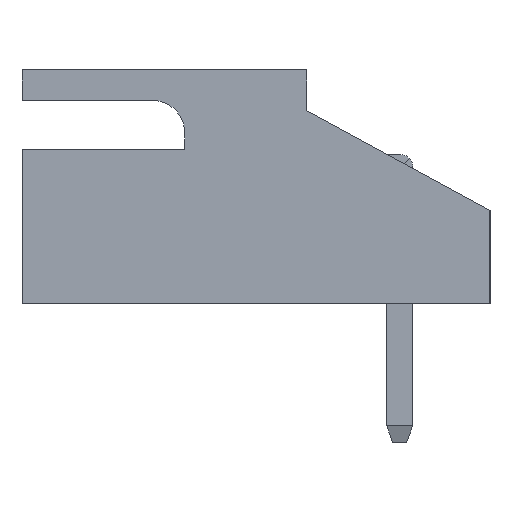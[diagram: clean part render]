
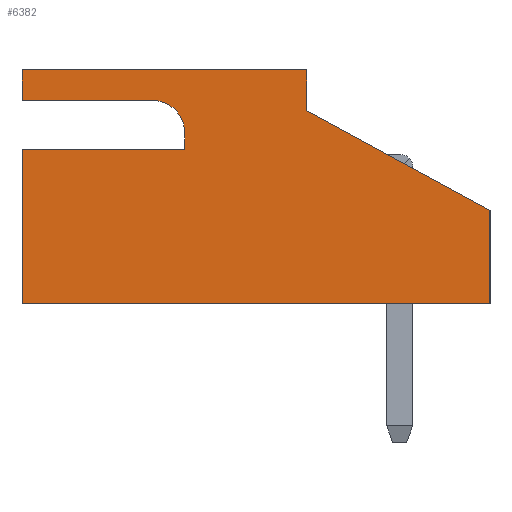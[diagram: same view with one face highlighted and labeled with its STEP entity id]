
A CAD part, left-side view. The second image highlights one B-rep face of the part: STEP entity #6382.
In plain terms, the highlighted planar face has unit normal (-1, 0, 0).
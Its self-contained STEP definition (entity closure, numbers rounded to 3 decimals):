
#104 = LINE ( 'NONE', #4746, #4784 ) ;
#234 = ORIENTED_EDGE ( 'NONE', *, *, #6420, .F. ) ;
#254 = LINE ( 'NONE', #6606, #1631 ) ;
#255 = VERTEX_POINT ( 'NONE', #4761 ) ;
#322 = ORIENTED_EDGE ( 'NONE', *, *, #5219, .T. ) ;
#358 = CARTESIAN_POINT ( 'NONE',  ( -16.25, 7., 0.925 ) ) ;
#362 = LINE ( 'NONE', #5617, #2933 ) ;
#395 = DIRECTION ( 'NONE',  ( 0., 0., -1. ) ) ;
#410 = DIRECTION ( 'NONE',  ( 1., 0., 0. ) ) ;
#445 = CARTESIAN_POINT ( 'NONE',  ( -16.25, 3.8, 1.325 ) ) ;
#536 = LINE ( 'NONE', #4723, #3891 ) ;
#648 = EDGE_CURVE ( 'NONE', #5474, #1851, #536, .T. ) ;
#1144 = CARTESIAN_POINT ( 'NONE',  ( -16.25, 7., 2.875 ) ) ;
#1180 = CARTESIAN_POINT ( 'NONE',  ( -16.25, 3., 0.925 ) ) ;
#1228 = VECTOR ( 'NONE', #1668, 1000. ) ;
#1345 = VERTEX_POINT ( 'NONE', #1497 ) ;
#1456 = LINE ( 'NONE', #6197, #3584 ) ;
#1497 = CARTESIAN_POINT ( 'NONE',  ( -16.25, 3.8, 2.125 ) ) ;
#1550 = VERTEX_POINT ( 'NONE', #6348 ) ;
#1580 = LINE ( 'NONE', #1144, #6653 ) ;
#1631 = VECTOR ( 'NONE', #3945, 1000. ) ;
#1638 = VERTEX_POINT ( 'NONE', #5512 ) ;
#1664 = VERTEX_POINT ( 'NONE', #4373 ) ;
#1668 = DIRECTION ( 'NONE',  ( 0., -1., 0. ) ) ;
#1678 = LINE ( 'NONE', #5910, #5252 ) ;
#1747 = FACE_OUTER_BOUND ( 'NONE', #6613, .T. ) ;
#1822 = ORIENTED_EDGE ( 'NONE', *, *, #5441, .T. ) ;
#1851 = VERTEX_POINT ( 'NONE', #358 ) ;
#1900 = ORIENTED_EDGE ( 'NONE', *, *, #648, .T. ) ;
#2070 = DIRECTION ( 'NONE',  ( 0., 0., 1. ) ) ;
#2105 = CARTESIAN_POINT ( 'NONE',  ( -16.25, 0., -2.875 ) ) ;
#2110 = DIRECTION ( 'NONE',  ( 0., 1., 0. ) ) ;
#2175 = DIRECTION ( 'NONE',  ( 0., 0., 1. ) ) ;
#2222 = DIRECTION ( 'NONE',  ( 0., 0., -1. ) ) ;
#2363 = CIRCLE ( 'NONE', #2586, 0.8 ) ;
#2400 = EDGE_CURVE ( 'NONE', #1664, #1851, #104, .T. ) ;
#2419 = DIRECTION ( 'NONE',  ( 0., 0., -1. ) ) ;
#2432 = ORIENTED_EDGE ( 'NONE', *, *, #4714, .F. ) ;
#2586 = AXIS2_PLACEMENT_3D ( 'NONE', #445, #410, #2419 ) ;
#2593 = ORIENTED_EDGE ( 'NONE', *, *, #3052, .F. ) ;
#2684 = CARTESIAN_POINT ( 'NONE',  ( -16.25, 7., -2.875 ) ) ;
#2700 = CARTESIAN_POINT ( 'NONE',  ( -16.25, 7., -2.875 ) ) ;
#2709 = DIRECTION ( 'NONE',  ( 0., 0., -1. ) ) ;
#2710 = LINE ( 'NONE', #2105, #4760 ) ;
#2933 = VECTOR ( 'NONE', #395, 1000. ) ;
#3036 = CARTESIAN_POINT ( 'NONE',  ( -16.25, 0., 2.875 ) ) ;
#3052 = EDGE_CURVE ( 'NONE', #255, #5594, #254, .T. ) ;
#3114 = ORIENTED_EDGE ( 'NONE', *, *, #2400, .F. ) ;
#3283 = DIRECTION ( 'NONE',  ( 0., -0.878, -0.478 ) ) ;
#3291 = LINE ( 'NONE', #5399, #4542 ) ;
#3377 = ORIENTED_EDGE ( 'NONE', *, *, #4100, .T. ) ;
#3414 = CARTESIAN_POINT ( 'NONE',  ( -16.25, -4.5, -0.575 ) ) ;
#3584 = VECTOR ( 'NONE', #6747, 1000. ) ;
#3891 = VECTOR ( 'NONE', #2110, 1000. ) ;
#3945 = DIRECTION ( 'NONE',  ( 0., 0., 1. ) ) ;
#4035 = ORIENTED_EDGE ( 'NONE', *, *, #4210, .F. ) ;
#4053 = CARTESIAN_POINT ( 'NONE',  ( -16.25, 3., 1.325 ) ) ;
#4100 = EDGE_CURVE ( 'NONE', #1345, #4350, #2363, .T. ) ;
#4210 = EDGE_CURVE ( 'NONE', #5594, #6644, #1580, .T. ) ;
#4350 = VERTEX_POINT ( 'NONE', #4053 ) ;
#4373 = CARTESIAN_POINT ( 'NONE',  ( -16.25, 7., -2.875 ) ) ;
#4542 = VECTOR ( 'NONE', #2709, 1000. ) ;
#4551 = ORIENTED_EDGE ( 'NONE', *, *, #5823, .T. ) ;
#4714 = EDGE_CURVE ( 'NONE', #6540, #1638, #3291, .T. ) ;
#4723 = CARTESIAN_POINT ( 'NONE',  ( -16.25, 7., 0.925 ) ) ;
#4746 = CARTESIAN_POINT ( 'NONE',  ( -16.25, 7., -2.875 ) ) ;
#4760 = VECTOR ( 'NONE', #2175, 1000. ) ;
#4761 = CARTESIAN_POINT ( 'NONE',  ( -16.25, 7., 2.125 ) ) ;
#4784 = VECTOR ( 'NONE', #2070, 1000. ) ;
#4836 = DIRECTION ( 'NONE',  ( 1., 0., 0. ) ) ;
#4867 = PLANE ( 'NONE',  #4907 ) ;
#4907 = AXIS2_PLACEMENT_3D ( 'NONE', #2700, #4836, #2222 ) ;
#5219 = EDGE_CURVE ( 'NONE', #255, #1345, #1456, .T. ) ;
#5252 = VECTOR ( 'NONE', #3283, 1000. ) ;
#5285 = EDGE_CURVE ( 'NONE', #4350, #5474, #362, .T. ) ;
#5399 = CARTESIAN_POINT ( 'NONE',  ( -16.25, -4.5, -0.575 ) ) ;
#5441 = EDGE_CURVE ( 'NONE', #1664, #1638, #6343, .T. ) ;
#5474 = VERTEX_POINT ( 'NONE', #1180 ) ;
#5512 = CARTESIAN_POINT ( 'NONE',  ( -16.25, -4.5, -2.875 ) ) ;
#5594 = VERTEX_POINT ( 'NONE', #6437 ) ;
#5617 = CARTESIAN_POINT ( 'NONE',  ( -16.25, 3., 1.325 ) ) ;
#5823 = EDGE_CURVE ( 'NONE', #1550, #6644, #2710, .T. ) ;
#5910 = CARTESIAN_POINT ( 'NONE',  ( -16.25, 0., 1.875 ) ) ;
#6197 = CARTESIAN_POINT ( 'NONE',  ( -16.25, 7., 2.125 ) ) ;
#6255 = DIRECTION ( 'NONE',  ( 0., -1., 0. ) ) ;
#6343 = LINE ( 'NONE', #2684, #1228 ) ;
#6348 = CARTESIAN_POINT ( 'NONE',  ( -16.25, 0., 1.875 ) ) ;
#6351 = ORIENTED_EDGE ( 'NONE', *, *, #5285, .T. ) ;
#6382 = ADVANCED_FACE ( 'NONE', ( #1747 ), #4867, .F. ) ;
#6420 = EDGE_CURVE ( 'NONE', #1550, #6540, #1678, .T. ) ;
#6437 = CARTESIAN_POINT ( 'NONE',  ( -16.25, 7., 2.875 ) ) ;
#6540 = VERTEX_POINT ( 'NONE', #3414 ) ;
#6606 = CARTESIAN_POINT ( 'NONE',  ( -16.25, 7., -2.875 ) ) ;
#6613 = EDGE_LOOP ( 'NONE', ( #2593, #322, #3377, #6351, #1900, #3114, #1822, #2432, #234, #4551, #4035 ) ) ;
#6644 = VERTEX_POINT ( 'NONE', #3036 ) ;
#6653 = VECTOR ( 'NONE', #6255, 1000. ) ;
#6747 = DIRECTION ( 'NONE',  ( 0., -1., 0. ) ) ;
